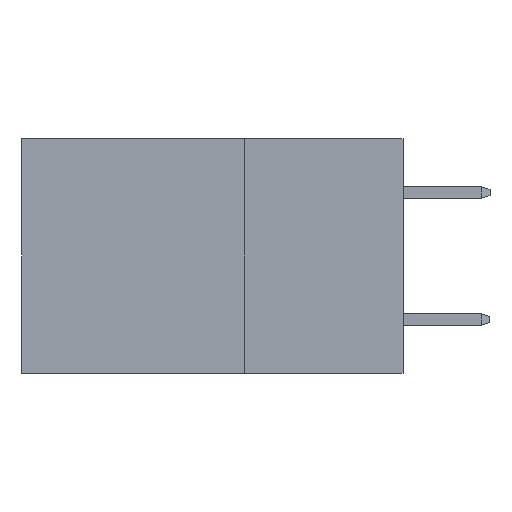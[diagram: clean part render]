
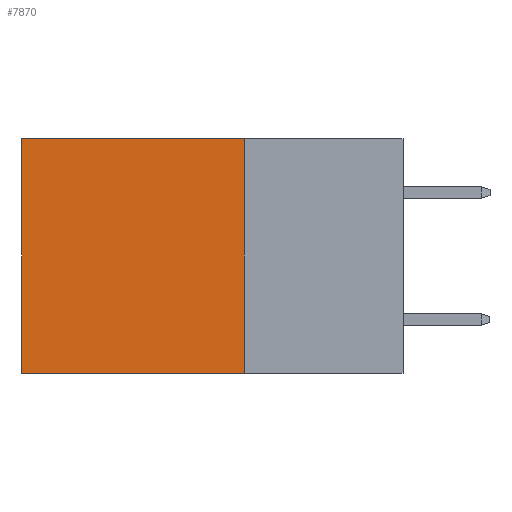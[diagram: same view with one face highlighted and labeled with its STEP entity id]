
A CAD part, left-side view. The second image highlights one B-rep face of the part: STEP entity #7870.
In plain terms, the highlighted planar face has unit normal (-1, 0, 0).
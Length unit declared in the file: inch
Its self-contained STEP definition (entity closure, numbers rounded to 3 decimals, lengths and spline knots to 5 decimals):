
#50 = ORIENTED_EDGE ( 'NONE', *, *, #3467, .T. ) ;
#1097 = CARTESIAN_POINT ( 'NONE',  ( 0.2875, 0.25, 0. ) ) ;
#1311 = VECTOR ( 'NONE', #2827, 39.37008 ) ;
#1372 = LINE ( 'NONE', #10445, #9478 ) ;
#1549 = EDGE_CURVE ( 'NONE', #2971, #10947, #5300, .T. ) ;
#1569 = CARTESIAN_POINT ( 'NONE',  ( 0.2875, 0.6, 0. ) ) ;
#1614 = LINE ( 'NONE', #8255, #5240 ) ;
#1873 = ORIENTED_EDGE ( 'NONE', *, *, #10788, .F. ) ;
#2220 = AXIS2_PLACEMENT_3D ( 'NONE', #1097, #9505, #7735 ) ;
#2661 = VERTEX_POINT ( 'NONE', #5826 ) ;
#2689 = CARTESIAN_POINT ( 'NONE',  ( 0.2875, 0.6, -0.37 ) ) ;
#2827 = DIRECTION ( 'NONE',  ( 0., 1., 0. ) ) ;
#2882 = CARTESIAN_POINT ( 'NONE',  ( 0.2875, 0.25, -0.37 ) ) ;
#2971 = VERTEX_POINT ( 'NONE', #3947 ) ;
#3467 = EDGE_CURVE ( 'NONE', #10947, #4719, #1372, .T. ) ;
#3947 = CARTESIAN_POINT ( 'NONE',  ( 0.2875, 0.25, 0. ) ) ;
#4566 = EDGE_CURVE ( 'NONE', #2971, #2661, #1614, .T. ) ;
#4719 = VERTEX_POINT ( 'NONE', #2689 ) ;
#5240 = VECTOR ( 'NONE', #10855, 39.37008 ) ;
#5245 = CARTESIAN_POINT ( 'NONE',  ( 0.2875, 0.25, 0. ) ) ;
#5300 = LINE ( 'NONE', #5245, #1311 ) ;
#5826 = CARTESIAN_POINT ( 'NONE',  ( 0.2875, 0.25, -0.37 ) ) ;
#6223 = DIRECTION ( 'NONE',  ( 0., 0., -1. ) ) ;
#6818 = ORIENTED_EDGE ( 'NONE', *, *, #4566, .F. ) ;
#7735 = DIRECTION ( 'NONE',  ( 0., 0., -1. ) ) ;
#7870 = ADVANCED_FACE ( 'NONE', ( #10335 ), #10511, .F. ) ;
#8019 = VECTOR ( 'NONE', #10587, 39.37008 ) ;
#8255 = CARTESIAN_POINT ( 'NONE',  ( 0.2875, 0.25, 0. ) ) ;
#8969 = LINE ( 'NONE', #2882, #8019 ) ;
#9478 = VECTOR ( 'NONE', #6223, 39.37008 ) ;
#9505 = DIRECTION ( 'NONE',  ( 1., 0., 0. ) ) ;
#9528 = ORIENTED_EDGE ( 'NONE', *, *, #1549, .T. ) ;
#9866 = EDGE_LOOP ( 'NONE', ( #50, #1873, #6818, #9528 ) ) ;
#10335 = FACE_OUTER_BOUND ( 'NONE', #9866, .T. ) ;
#10445 = CARTESIAN_POINT ( 'NONE',  ( 0.2875, 0.6, 0. ) ) ;
#10511 = PLANE ( 'NONE',  #2220 ) ;
#10587 = DIRECTION ( 'NONE',  ( 0., 1., 0. ) ) ;
#10788 = EDGE_CURVE ( 'NONE', #2661, #4719, #8969, .T. ) ;
#10855 = DIRECTION ( 'NONE',  ( 0., 0., -1. ) ) ;
#10947 = VERTEX_POINT ( 'NONE', #1569 ) ;
